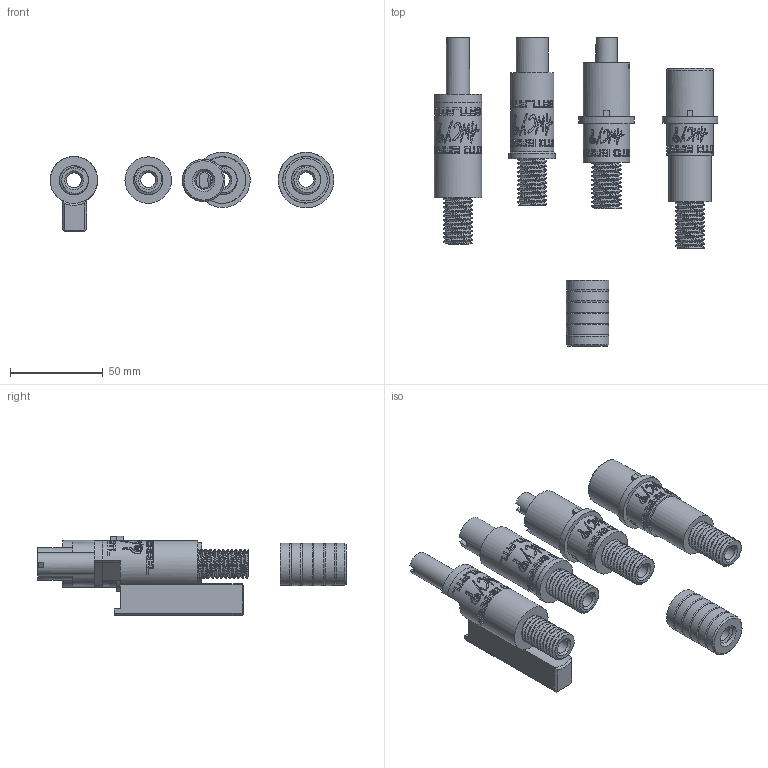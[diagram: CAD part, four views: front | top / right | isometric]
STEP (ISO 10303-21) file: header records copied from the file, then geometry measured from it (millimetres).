
FILE_DESCRIPTION(/* description */ (''),/* implementation_level */ '2;1');
FILE_NAME(/* name */ 'Proto Barrel RC1 v75.step',/* time_stamp */ '2022-01-09T10:22:02-05:00',/* author */ (''),/* organization */ (''),/* preprocessor_version */ 'ST-DEVELOPER v18.1',/* originating_system */ 'Autodesk Translation Framework v10.10.0.1391',/* authorisation */ '');
FILE_SCHEMA (('AUTOMOTIVE_DESIGN { 1 0 10303 214 3 1 1 }'));
Products named in the file (3): Proto Barrel RC1; Proto Barrel Parts; Gatlatl Breech Retainers
Assembly tree (2 placements, depth 3):
  Proto Barrel RC1
    Proto Barrel Parts
      Gatlatl Breech Retainers
Bounding box: 152.67 x 166.29 x 42.96 mm (x, y, z)
Volume: 127625.4 mm3; surface area: 55210.9 mm2
Topology: 5 solids, 6 shells, 3055 faces, 8633 edges, 5742 vertices
Faces by surface type: bspline 1917, plane 809, cylinder 308, cone 11, torus 10
Full cylindrical faces by diameter (mm): 2 x1, 4 x1, 7 x1, 8.1 x5, 8.2 x1, 8.4 x1, 11.4 x1, 12.5 x1, 13.086 x10, 13.127 x30, 13.541 x10, 15 x1, 15.603 x10, 15.723 x30, 15.875 x10, 17.44 x1, 21.291 x1, 22.8 x7, 23.368 x1, 25 x3, 25.222 x2, 29.845 x2
Entity records: 148107 total; most frequent: CARTESIAN_POINT 83653, ORIENTED_EDGE 17266, EDGE_CURVE 8633, DIRECTION 6567, VERTEX_POINT 5742, B_SPLINE_CURVE_WITH_KNOTS 4831, LINE 3313, VECTOR 3313
